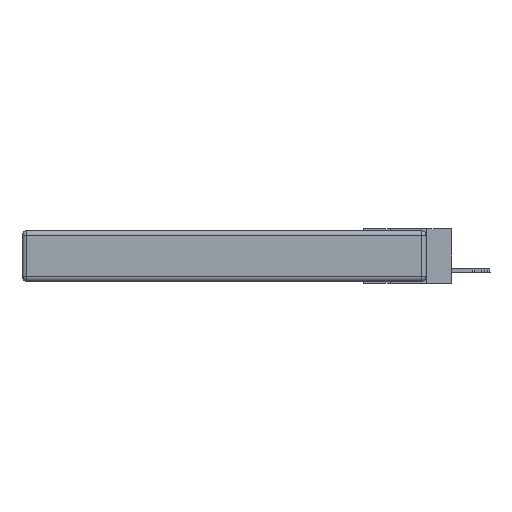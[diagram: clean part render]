
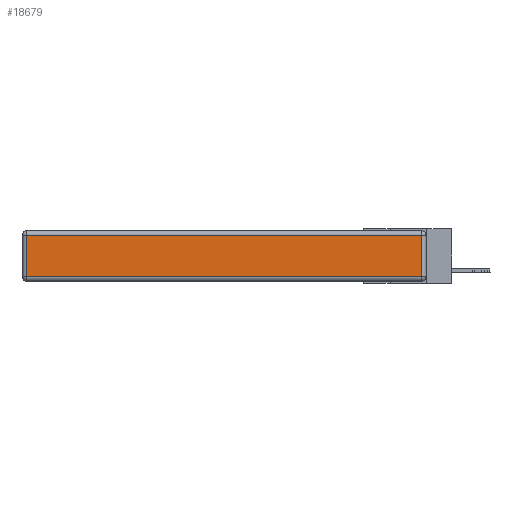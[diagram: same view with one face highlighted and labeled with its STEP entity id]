
A CAD part, left-side view. The second image highlights one B-rep face of the part: STEP entity #18679.
In plain terms, the highlighted planar face has unit normal (-1, 0, 0).
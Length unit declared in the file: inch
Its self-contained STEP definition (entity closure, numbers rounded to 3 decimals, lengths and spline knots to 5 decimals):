
#1120 = EDGE_CURVE ( 'NONE', #16255, #10475, #21516, .T. ) ;
#1292 = CARTESIAN_POINT ( 'NONE',  ( 0., 2.72, -0.343 ) ) ;
#2191 = VECTOR ( 'NONE', #21888, 39.37008 ) ;
#2677 = EDGE_CURVE ( 'NONE', #26884, #20885, #19222, .T. ) ;
#3030 = DIRECTION ( 'NONE',  ( 0., 0., 1. ) ) ;
#7930 = DIRECTION ( 'NONE',  ( 0., 0., -1. ) ) ;
#8532 = EDGE_CURVE ( 'NONE', #10475, #26884, #12940, .T. ) ;
#8841 = CARTESIAN_POINT ( 'NONE',  ( 0., 0., -0.313 ) ) ;
#9212 = VECTOR ( 'NONE', #12066, 39.37008 ) ;
#9585 = CARTESIAN_POINT ( 'NONE',  ( 0., 2.75, -0.03 ) ) ;
#9904 = FACE_OUTER_BOUND ( 'NONE', #27731, .T. ) ;
#10475 = VERTEX_POINT ( 'NONE', #28607 ) ;
#12066 = DIRECTION ( 'NONE',  ( 0., 1., 0. ) ) ;
#12933 = CARTESIAN_POINT ( 'NONE',  ( 0., 0.03, -0.03 ) ) ;
#12940 = LINE ( 'NONE', #17075, #2191 ) ;
#13233 = VECTOR ( 'NONE', #22918, 39.37008 ) ;
#14548 = AXIS2_PLACEMENT_3D ( 'NONE', #14677, #23645, #3030 ) ;
#14677 = CARTESIAN_POINT ( 'NONE',  ( 0., 0., -0.343 ) ) ;
#15774 = LINE ( 'NONE', #1292, #28721 ) ;
#16255 = VERTEX_POINT ( 'NONE', #19467 ) ;
#16586 = EDGE_CURVE ( 'NONE', #20885, #16255, #15774, .T. ) ;
#17075 = CARTESIAN_POINT ( 'NONE',  ( 0., 0.03, -0.343 ) ) ;
#18679 = ADVANCED_FACE ( 'NONE', ( #9904 ), #25873, .T. ) ;
#18803 = ORIENTED_EDGE ( 'NONE', *, *, #8532, .T. ) ;
#19222 = LINE ( 'NONE', #9585, #9212 ) ;
#19467 = CARTESIAN_POINT ( 'NONE',  ( 0., 2.72, -0.313 ) ) ;
#20885 = VERTEX_POINT ( 'NONE', #23840 ) ;
#21516 = LINE ( 'NONE', #8841, #13233 ) ;
#21888 = DIRECTION ( 'NONE',  ( 0., 0., 1. ) ) ;
#22918 = DIRECTION ( 'NONE',  ( 0., -1., 0. ) ) ;
#23645 = DIRECTION ( 'NONE',  ( -1., 0., 0. ) ) ;
#23840 = CARTESIAN_POINT ( 'NONE',  ( 0., 2.72, -0.03 ) ) ;
#24931 = ORIENTED_EDGE ( 'NONE', *, *, #2677, .T. ) ;
#25873 = PLANE ( 'NONE',  #14548 ) ;
#26884 = VERTEX_POINT ( 'NONE', #12933 ) ;
#26922 = ORIENTED_EDGE ( 'NONE', *, *, #16586, .T. ) ;
#27731 = EDGE_LOOP ( 'NONE', ( #29415, #18803, #24931, #26922 ) ) ;
#28607 = CARTESIAN_POINT ( 'NONE',  ( 0., 0.03, -0.313 ) ) ;
#28721 = VECTOR ( 'NONE', #7930, 39.37008 ) ;
#29415 = ORIENTED_EDGE ( 'NONE', *, *, #1120, .T. ) ;
